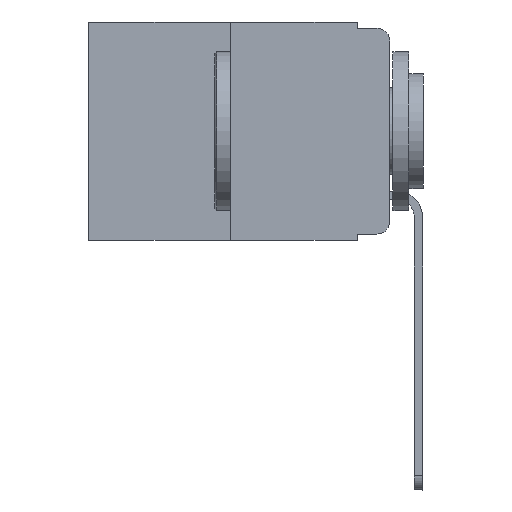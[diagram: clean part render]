
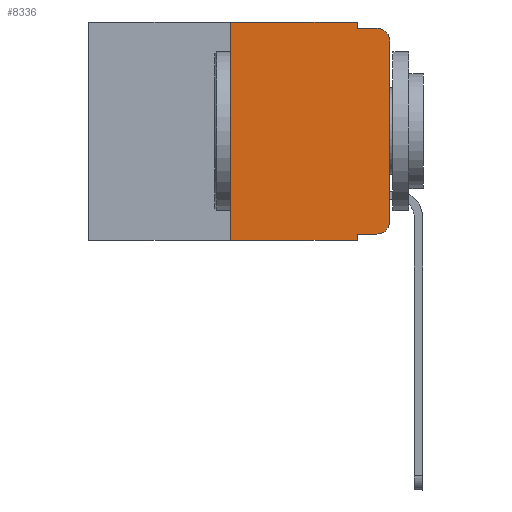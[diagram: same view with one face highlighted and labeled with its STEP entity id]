
A CAD part, left-side view. The second image highlights one B-rep face of the part: STEP entity #8336.
In plain terms, the highlighted planar face has unit normal (-1, 0, 0).
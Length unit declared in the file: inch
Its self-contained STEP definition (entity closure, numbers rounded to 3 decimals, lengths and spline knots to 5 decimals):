
#804 = CARTESIAN_POINT ( 'NONE',  ( 0., 0.473, 0. ) ) ;
#844 = CARTESIAN_POINT ( 'NONE',  ( 0., 0.473, -0.343 ) ) ;
#1306 = VECTOR ( 'NONE', #22646, 39.37008 ) ;
#2014 = ORIENTED_EDGE ( 'NONE', *, *, #11105, .T. ) ;
#2258 = VERTEX_POINT ( 'NONE', #13499 ) ;
#2469 = CARTESIAN_POINT ( 'NONE',  ( 0., 0.051, 0. ) ) ;
#2489 = DIRECTION ( 'NONE',  ( 0., -1., 0. ) ) ;
#2606 = DIRECTION ( 'NONE',  ( 0., 0., -1. ) ) ;
#2802 = ORIENTED_EDGE ( 'NONE', *, *, #24475, .T. ) ;
#2862 = LINE ( 'NONE', #10934, #4250 ) ;
#3192 = CARTESIAN_POINT ( 'NONE',  ( 0., 0.25, 0. ) ) ;
#3566 = CARTESIAN_POINT ( 'NONE',  ( 0., 0.051, 0. ) ) ;
#4250 = VECTOR ( 'NONE', #8950, 39.37008 ) ;
#4423 = DIRECTION ( 'NONE',  ( 0., 0., -1. ) ) ;
#5357 = DIRECTION ( 'NONE',  ( 0., 0., -1. ) ) ;
#6072 = ORIENTED_EDGE ( 'NONE', *, *, #12026, .F. ) ;
#6399 = CARTESIAN_POINT ( 'NONE',  ( 0., 0.02, -0.313 ) ) ;
#6445 = CARTESIAN_POINT ( 'NONE',  ( 0., 0.051, -0.01 ) ) ;
#6831 = AXIS2_PLACEMENT_3D ( 'NONE', #13968, #15969, #5357 ) ;
#7473 = AXIS2_PLACEMENT_3D ( 'NONE', #804, #15114, #20820 ) ;
#7913 = ORIENTED_EDGE ( 'NONE', *, *, #23526, .F. ) ;
#8061 = CARTESIAN_POINT ( 'NONE',  ( 0., 0.051, -0.01 ) ) ;
#8336 = ADVANCED_FACE ( 'NONE', ( #10595 ), #9010, .F. ) ;
#8485 = VECTOR ( 'NONE', #2606, 39.37008 ) ;
#8516 = VERTEX_POINT ( 'NONE', #3566 ) ;
#8950 = DIRECTION ( 'NONE',  ( 0., -1., 0. ) ) ;
#8970 = VERTEX_POINT ( 'NONE', #17748 ) ;
#9010 = PLANE ( 'NONE',  #7473 ) ;
#9161 = VERTEX_POINT ( 'NONE', #20382 ) ;
#9320 = LINE ( 'NONE', #21002, #21490 ) ;
#9899 = ORIENTED_EDGE ( 'NONE', *, *, #13951, .F. ) ;
#10014 = CARTESIAN_POINT ( 'NONE',  ( 0., 0.25, 0. ) ) ;
#10283 = DIRECTION ( 'NONE',  ( 0., 0., 1. ) ) ;
#10595 = FACE_OUTER_BOUND ( 'NONE', #20019, .T. ) ;
#10934 = CARTESIAN_POINT ( 'NONE',  ( 0., 0.473, 0. ) ) ;
#11105 = EDGE_CURVE ( 'NONE', #25357, #9161, #22571, .T. ) ;
#11538 = CARTESIAN_POINT ( 'NONE',  ( 0., 0.02, -0.333 ) ) ;
#12026 = EDGE_CURVE ( 'NONE', #22149, #2258, #24626, .T. ) ;
#12205 = ORIENTED_EDGE ( 'NONE', *, *, #17855, .T. ) ;
#12562 = CARTESIAN_POINT ( 'NONE',  ( 0., 0.051, 0. ) ) ;
#12763 = CIRCLE ( 'NONE', #6831, 0.02 ) ;
#13174 = CIRCLE ( 'NONE', #19949, 0.02 ) ;
#13499 = CARTESIAN_POINT ( 'NONE',  ( 0., 0.02, -0.01 ) ) ;
#13951 = EDGE_CURVE ( 'NONE', #23306, #8516, #2862, .T. ) ;
#13968 = CARTESIAN_POINT ( 'NONE',  ( 0., 0.02, -0.03 ) ) ;
#14506 = DIRECTION ( 'NONE',  ( -1., 0., 0. ) ) ;
#14587 = CARTESIAN_POINT ( 'NONE',  ( 0., 0., -0.03 ) ) ;
#14595 = ORIENTED_EDGE ( 'NONE', *, *, #24060, .F. ) ;
#14965 = LINE ( 'NONE', #12562, #1306 ) ;
#15114 = DIRECTION ( 'NONE',  ( 1., 0., 0. ) ) ;
#15296 = VECTOR ( 'NONE', #21005, 39.37008 ) ;
#15562 = EDGE_CURVE ( 'NONE', #25357, #23306, #18123, .T. ) ;
#15649 = LINE ( 'NONE', #17170, #15296 ) ;
#15969 = DIRECTION ( 'NONE',  ( -1., 0., 0. ) ) ;
#16393 = ORIENTED_EDGE ( 'NONE', *, *, #24573, .T. ) ;
#17026 = CARTESIAN_POINT ( 'NONE',  ( 0., 0.25, -0.343 ) ) ;
#17041 = DIRECTION ( 'NONE',  ( 0., 0., 1. ) ) ;
#17170 = CARTESIAN_POINT ( 'NONE',  ( 0., 0.051, -0.333 ) ) ;
#17748 = CARTESIAN_POINT ( 'NONE',  ( 0., 0.051, -0.333 ) ) ;
#17855 = EDGE_CURVE ( 'NONE', #21633, #23097, #9320, .T. ) ;
#18123 = LINE ( 'NONE', #10014, #25626 ) ;
#18204 = ORIENTED_EDGE ( 'NONE', *, *, #15562, .F. ) ;
#18507 = LINE ( 'NONE', #2469, #8485 ) ;
#18999 = VECTOR ( 'NONE', #2489, 39.37008 ) ;
#19949 = AXIS2_PLACEMENT_3D ( 'NONE', #6399, #14506, #4423 ) ;
#20019 = EDGE_LOOP ( 'NONE', ( #12205, #21182, #6072, #14595, #9899, #18204, #2014, #7913, #16393, #2802 ) ) ;
#20167 = CARTESIAN_POINT ( 'NONE',  ( 0., 0., -0.313 ) ) ;
#20382 = CARTESIAN_POINT ( 'NONE',  ( 0., 0.051, -0.343 ) ) ;
#20820 = DIRECTION ( 'NONE',  ( 0., 0., -1. ) ) ;
#21002 = CARTESIAN_POINT ( 'NONE',  ( 0., 0., 0. ) ) ;
#21005 = DIRECTION ( 'NONE',  ( 0., -1., 0. ) ) ;
#21182 = ORIENTED_EDGE ( 'NONE', *, *, #25128, .T. ) ;
#21490 = VECTOR ( 'NONE', #17041, 39.37008 ) ;
#21633 = VERTEX_POINT ( 'NONE', #20167 ) ;
#21988 = VECTOR ( 'NONE', #25227, 39.37008 ) ;
#22149 = VERTEX_POINT ( 'NONE', #8061 ) ;
#22571 = LINE ( 'NONE', #844, #21988 ) ;
#22646 = DIRECTION ( 'NONE',  ( 0., 0., -1. ) ) ;
#23097 = VERTEX_POINT ( 'NONE', #14587 ) ;
#23306 = VERTEX_POINT ( 'NONE', #3192 ) ;
#23526 = EDGE_CURVE ( 'NONE', #8970, #9161, #14965, .T. ) ;
#24060 = EDGE_CURVE ( 'NONE', #8516, #22149, #18507, .T. ) ;
#24475 = EDGE_CURVE ( 'NONE', #24619, #21633, #13174, .T. ) ;
#24573 = EDGE_CURVE ( 'NONE', #8970, #24619, #15649, .T. ) ;
#24619 = VERTEX_POINT ( 'NONE', #11538 ) ;
#24626 = LINE ( 'NONE', #6445, #18999 ) ;
#25128 = EDGE_CURVE ( 'NONE', #23097, #2258, #12763, .T. ) ;
#25227 = DIRECTION ( 'NONE',  ( 0., -1., 0. ) ) ;
#25357 = VERTEX_POINT ( 'NONE', #17026 ) ;
#25626 = VECTOR ( 'NONE', #10283, 39.37008 ) ;
